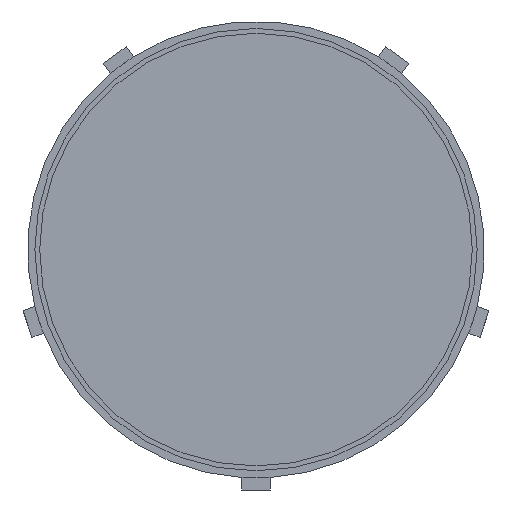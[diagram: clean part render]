
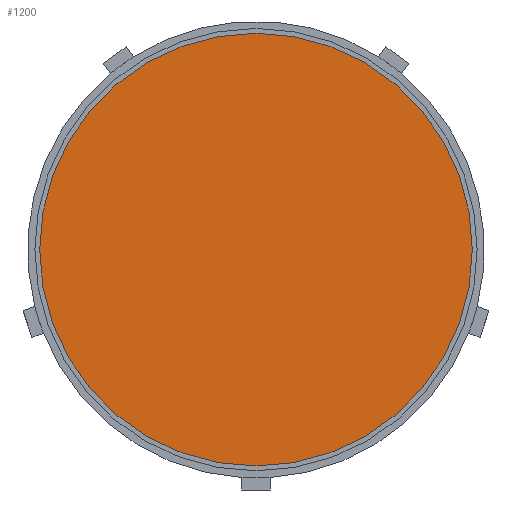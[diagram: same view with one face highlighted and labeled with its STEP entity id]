
A CAD part, front view. The second image highlights one B-rep face of the part: STEP entity #1200.
In plain terms, the highlighted planar face has unit normal (0, -1, 0).
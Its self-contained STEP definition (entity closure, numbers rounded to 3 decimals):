
#41 = AXIS2_PLACEMENT_3D ( 'NONE', #878, #1026, #183 ) ;
#116 = AXIS2_PLACEMENT_3D ( 'NONE', #391, #1414, #530 ) ;
#183 = DIRECTION ( 'NONE',  ( 0., 0., 1. ) ) ;
#391 = CARTESIAN_POINT ( 'NONE',  ( 0., 70., 0. ) ) ;
#440 = CARTESIAN_POINT ( 'NONE',  ( 0., 70., 0. ) ) ;
#481 = AXIS2_PLACEMENT_3D ( 'NONE', #440, #1465, #581 ) ;
#530 = DIRECTION ( 'NONE',  ( 0., 0., 1. ) ) ;
#544 = VERTEX_POINT ( 'NONE', #1229 ) ;
#553 = FACE_OUTER_BOUND ( 'NONE', #808, .T. ) ;
#581 = DIRECTION ( 'NONE',  ( 0., 0., 1. ) ) ;
#808 = EDGE_LOOP ( 'NONE', ( #1579, #1157 ) ) ;
#878 = CARTESIAN_POINT ( 'NONE',  ( 0., 70., 0. ) ) ;
#997 = EDGE_CURVE ( 'NONE', #544, #1607, #1710, .T. ) ;
#1026 = DIRECTION ( 'NONE',  ( 0., 1., 0. ) ) ;
#1157 = ORIENTED_EDGE ( 'NONE', *, *, #997, .F. ) ;
#1200 = ADVANCED_FACE ( 'NONE', ( #553 ), #1779, .F. ) ;
#1216 = CIRCLE ( 'NONE', #116, 90. ) ;
#1229 = CARTESIAN_POINT ( 'NONE',  ( 0., 70., 90. ) ) ;
#1414 = DIRECTION ( 'NONE',  ( 0., 1., 0. ) ) ;
#1431 = EDGE_CURVE ( 'NONE', #1607, #544, #1216, .T. ) ;
#1465 = DIRECTION ( 'NONE',  ( 0., 1., 0. ) ) ;
#1579 = ORIENTED_EDGE ( 'NONE', *, *, #1431, .F. ) ;
#1607 = VERTEX_POINT ( 'NONE', #1612 ) ;
#1612 = CARTESIAN_POINT ( 'NONE',  ( 0., 70., -90. ) ) ;
#1710 = CIRCLE ( 'NONE', #481, 90. ) ;
#1779 = PLANE ( 'NONE',  #41 ) ;
